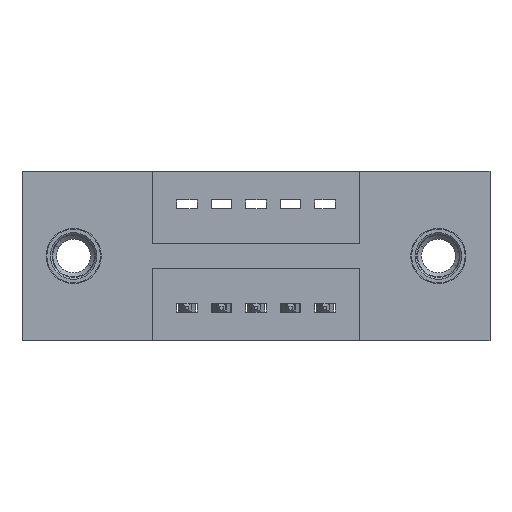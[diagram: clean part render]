
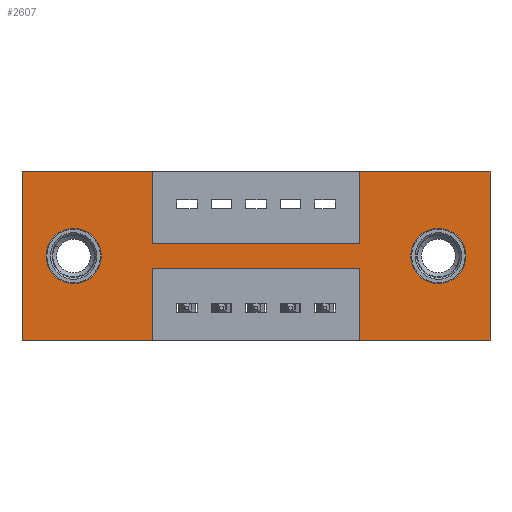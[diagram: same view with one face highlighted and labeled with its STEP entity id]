
A CAD part, front view. The second image highlights one B-rep face of the part: STEP entity #2607.
In plain terms, the highlighted planar face has unit normal (0, -1, 0).
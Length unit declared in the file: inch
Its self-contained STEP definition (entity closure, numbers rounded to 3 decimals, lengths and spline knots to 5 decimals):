
#157 = CARTESIAN_POINT ( 'NONE',  ( 0.1495, 0., -0.245 ) ) ;
#197 = DIRECTION ( 'NONE',  ( 1., 0., 0. ) ) ;
#203 = AXIS2_PLACEMENT_3D ( 'NONE', #157, #5057, #3657 ) ;
#248 = VECTOR ( 'NONE', #7604, 39.37008 ) ;
#286 = DIRECTION ( 'NONE',  ( 0., 0., -1. ) ) ;
#350 = EDGE_LOOP ( 'NONE', ( #7733, #8435, #835, #699, #1627, #6463, #6455, #4688, #6241, #8505, #3470, #5362 ) ) ;
#413 = EDGE_CURVE ( 'NONE', #2825, #4843, #7675, .T. ) ;
#619 = CARTESIAN_POINT ( 'NONE',  ( 0.3775, 0., -0.21 ) ) ;
#699 = ORIENTED_EDGE ( 'NONE', *, *, #1293, .F. ) ;
#725 = CARTESIAN_POINT ( 'NONE',  ( 0.3775, 0., -0.28 ) ) ;
#753 = CARTESIAN_POINT ( 'NONE',  ( 0., 0., 0. ) ) ;
#770 = DIRECTION ( 'NONE',  ( 0., 0., 1. ) ) ;
#835 = ORIENTED_EDGE ( 'NONE', *, *, #8266, .F. ) ;
#943 = DIRECTION ( 'NONE',  ( 0., 0., -1. ) ) ;
#1012 = VECTOR ( 'NONE', #1283, 39.37008 ) ;
#1149 = ORIENTED_EDGE ( 'NONE', *, *, #6094, .T. ) ;
#1283 = DIRECTION ( 'NONE',  ( 0., 0., -1. ) ) ;
#1293 = EDGE_CURVE ( 'NONE', #7186, #2283, #7111, .T. ) ;
#1465 = CIRCLE ( 'NONE', #5877, 0.08 ) ;
#1468 = FACE_BOUND ( 'NONE', #7034, .T. ) ;
#1577 = VERTEX_POINT ( 'NONE', #7844 ) ;
#1581 = FACE_BOUND ( 'NONE', #3711, .T. ) ;
#1608 = CARTESIAN_POINT ( 'NONE',  ( 0.3775, 0., 0. ) ) ;
#1627 = ORIENTED_EDGE ( 'NONE', *, *, #3113, .F. ) ;
#1644 = LINE ( 'NONE', #619, #4049 ) ;
#1812 = VECTOR ( 'NONE', #197, 39.37008 ) ;
#1910 = VECTOR ( 'NONE', #5036, 39.37008 ) ;
#1930 = AXIS2_PLACEMENT_3D ( 'NONE', #2100, #3488, #770 ) ;
#2018 = CARTESIAN_POINT ( 'NONE',  ( 1.2055, 0., -0.165 ) ) ;
#2030 = CARTESIAN_POINT ( 'NONE',  ( 0.9775, 0., -0.21 ) ) ;
#2049 = DIRECTION ( 'NONE',  ( 0., 0., -1. ) ) ;
#2100 = CARTESIAN_POINT ( 'NONE',  ( 0.1495, 0., -0.245 ) ) ;
#2242 = VECTOR ( 'NONE', #4327, 39.37008 ) ;
#2283 = VERTEX_POINT ( 'NONE', #1608 ) ;
#2378 = DIRECTION ( 'NONE',  ( 0., 0., 1. ) ) ;
#2573 = LINE ( 'NONE', #725, #2242 ) ;
#2589 = EDGE_CURVE ( 'NONE', #6761, #2830, #4214, .T. ) ;
#2607 = ADVANCED_FACE ( 'NONE', ( #1468, #1581, #5552 ), #3781, .T. ) ;
#2649 = VECTOR ( 'NONE', #5349, 39.37008 ) ;
#2789 = CARTESIAN_POINT ( 'NONE',  ( 0.1495, 0., -0.165 ) ) ;
#2804 = DIRECTION ( 'NONE',  ( -1., 0., 0. ) ) ;
#2825 = VERTEX_POINT ( 'NONE', #8966 ) ;
#2830 = VERTEX_POINT ( 'NONE', #4775 ) ;
#2859 = LINE ( 'NONE', #6645, #8335 ) ;
#2937 = CARTESIAN_POINT ( 'NONE',  ( 1.2055, 0., -0.325 ) ) ;
#2944 = EDGE_CURVE ( 'NONE', #4843, #2825, #4205, .T. ) ;
#2997 = VERTEX_POINT ( 'NONE', #4907 ) ;
#3080 = VECTOR ( 'NONE', #3163, 39.37008 ) ;
#3113 = EDGE_CURVE ( 'NONE', #1577, #7186, #7247, .T. ) ;
#3115 = CARTESIAN_POINT ( 'NONE',  ( 0.3775, 0., -0.21 ) ) ;
#3122 = CARTESIAN_POINT ( 'NONE',  ( 0.9775, 0., 0. ) ) ;
#3163 = DIRECTION ( 'NONE',  ( -1., 0., 0. ) ) ;
#3470 = ORIENTED_EDGE ( 'NONE', *, *, #3805, .F. ) ;
#3488 = DIRECTION ( 'NONE',  ( 0., 1., 0. ) ) ;
#3498 = EDGE_CURVE ( 'NONE', #4515, #8754, #4322, .T. ) ;
#3640 = CARTESIAN_POINT ( 'NONE',  ( 0.3775, 0., -0.49 ) ) ;
#3649 = CARTESIAN_POINT ( 'NONE',  ( 1.355, 0., 0. ) ) ;
#3657 = DIRECTION ( 'NONE',  ( 0., 0., 1. ) ) ;
#3690 = EDGE_CURVE ( 'NONE', #2997, #7426, #2573, .T. ) ;
#3711 = EDGE_LOOP ( 'NONE', ( #3800, #4841 ) ) ;
#3759 = CIRCLE ( 'NONE', #8379, 0.08 ) ;
#3781 = PLANE ( 'NONE',  #7533 ) ;
#3800 = ORIENTED_EDGE ( 'NONE', *, *, #2944, .T. ) ;
#3805 = EDGE_CURVE ( 'NONE', #8754, #5808, #9011, .T. ) ;
#4028 = CARTESIAN_POINT ( 'NONE',  ( 0.9775, 0., -0.49 ) ) ;
#4033 = EDGE_CURVE ( 'NONE', #6139, #8283, #3759, .T. ) ;
#4049 = VECTOR ( 'NONE', #7643, 39.37008 ) ;
#4069 = VECTOR ( 'NONE', #2804, 39.37008 ) ;
#4129 = EDGE_CURVE ( 'NONE', #2830, #4515, #6167, .T. ) ;
#4205 = CIRCLE ( 'NONE', #1930, 0.08 ) ;
#4214 = LINE ( 'NONE', #5233, #1812 ) ;
#4322 = LINE ( 'NONE', #4765, #8571 ) ;
#4327 = DIRECTION ( 'NONE',  ( -1., 0., 0. ) ) ;
#4515 = VERTEX_POINT ( 'NONE', #3122 ) ;
#4688 = ORIENTED_EDGE ( 'NONE', *, *, #3690, .F. ) ;
#4765 = CARTESIAN_POINT ( 'NONE',  ( 0., 0., 0. ) ) ;
#4775 = CARTESIAN_POINT ( 'NONE',  ( 0.9775, 0., -0.21 ) ) ;
#4841 = ORIENTED_EDGE ( 'NONE', *, *, #413, .T. ) ;
#4843 = VERTEX_POINT ( 'NONE', #2789 ) ;
#4907 = CARTESIAN_POINT ( 'NONE',  ( 0.9775, 0., -0.28 ) ) ;
#4957 = LINE ( 'NONE', #8681, #3080 ) ;
#4972 = EDGE_CURVE ( 'NONE', #5808, #8410, #7332, .T. ) ;
#5036 = DIRECTION ( 'NONE',  ( 0., 0., 1. ) ) ;
#5057 = DIRECTION ( 'NONE',  ( 0., 1., 0. ) ) ;
#5233 = CARTESIAN_POINT ( 'NONE',  ( 0.3775, 0., -0.21 ) ) ;
#5312 = VECTOR ( 'NONE', #943, 39.37008 ) ;
#5349 = DIRECTION ( 'NONE',  ( 1., 0., 0. ) ) ;
#5362 = ORIENTED_EDGE ( 'NONE', *, *, #3498, .F. ) ;
#5378 = CARTESIAN_POINT ( 'NONE',  ( 0., 0., 0. ) ) ;
#5457 = CARTESIAN_POINT ( 'NONE',  ( 1.2055, 0., -0.245 ) ) ;
#5552 = FACE_OUTER_BOUND ( 'NONE', #350, .T. ) ;
#5719 = LINE ( 'NONE', #6855, #1012 ) ;
#5769 = CARTESIAN_POINT ( 'NONE',  ( 1.2055, 0., -0.245 ) ) ;
#5808 = VERTEX_POINT ( 'NONE', #7603 ) ;
#5877 = AXIS2_PLACEMENT_3D ( 'NONE', #5769, #8545, #8597 ) ;
#6094 = EDGE_CURVE ( 'NONE', #8283, #6139, #1465, .T. ) ;
#6139 = VERTEX_POINT ( 'NONE', #2937 ) ;
#6167 = LINE ( 'NONE', #2030, #248 ) ;
#6241 = ORIENTED_EDGE ( 'NONE', *, *, #8796, .F. ) ;
#6242 = DIRECTION ( 'NONE',  ( 1., 0., 0. ) ) ;
#6310 = CARTESIAN_POINT ( 'NONE',  ( 0., 0., -0.49 ) ) ;
#6455 = ORIENTED_EDGE ( 'NONE', *, *, #7073, .F. ) ;
#6460 = CARTESIAN_POINT ( 'NONE',  ( 0., 0., 0. ) ) ;
#6463 = ORIENTED_EDGE ( 'NONE', *, *, #7377, .F. ) ;
#6569 = CARTESIAN_POINT ( 'NONE',  ( 1.355, 0., 0. ) ) ;
#6645 = CARTESIAN_POINT ( 'NONE',  ( 0.9775, 0., -0.28 ) ) ;
#6692 = VERTEX_POINT ( 'NONE', #3640 ) ;
#6761 = VERTEX_POINT ( 'NONE', #3115 ) ;
#6855 = CARTESIAN_POINT ( 'NONE',  ( 0.3775, 0., -0.28 ) ) ;
#7034 = EDGE_LOOP ( 'NONE', ( #1149, #8295 ) ) ;
#7073 = EDGE_CURVE ( 'NONE', #7426, #6692, #5719, .T. ) ;
#7111 = LINE ( 'NONE', #5378, #2649 ) ;
#7186 = VERTEX_POINT ( 'NONE', #753 ) ;
#7247 = LINE ( 'NONE', #6460, #1910 ) ;
#7312 = CARTESIAN_POINT ( 'NONE',  ( 0., 0., -0.49 ) ) ;
#7332 = LINE ( 'NONE', #6310, #4069 ) ;
#7377 = EDGE_CURVE ( 'NONE', #6692, #1577, #4957, .T. ) ;
#7426 = VERTEX_POINT ( 'NONE', #8849 ) ;
#7533 = AXIS2_PLACEMENT_3D ( 'NONE', #7312, #8031, #286 ) ;
#7603 = CARTESIAN_POINT ( 'NONE',  ( 1.355, 0., -0.49 ) ) ;
#7604 = DIRECTION ( 'NONE',  ( 0., 0., 1. ) ) ;
#7643 = DIRECTION ( 'NONE',  ( 0., 0., -1. ) ) ;
#7675 = CIRCLE ( 'NONE', #203, 0.08 ) ;
#7733 = ORIENTED_EDGE ( 'NONE', *, *, #4129, .F. ) ;
#7844 = CARTESIAN_POINT ( 'NONE',  ( 0., 0., -0.49 ) ) ;
#8031 = DIRECTION ( 'NONE',  ( 0., -1., 0. ) ) ;
#8266 = EDGE_CURVE ( 'NONE', #2283, #6761, #1644, .T. ) ;
#8283 = VERTEX_POINT ( 'NONE', #2018 ) ;
#8295 = ORIENTED_EDGE ( 'NONE', *, *, #4033, .T. ) ;
#8335 = VECTOR ( 'NONE', #2378, 39.37008 ) ;
#8379 = AXIS2_PLACEMENT_3D ( 'NONE', #5457, #9013, #2049 ) ;
#8410 = VERTEX_POINT ( 'NONE', #4028 ) ;
#8435 = ORIENTED_EDGE ( 'NONE', *, *, #2589, .F. ) ;
#8505 = ORIENTED_EDGE ( 'NONE', *, *, #4972, .F. ) ;
#8545 = DIRECTION ( 'NONE',  ( 0., 1., 0. ) ) ;
#8571 = VECTOR ( 'NONE', #6242, 39.37008 ) ;
#8597 = DIRECTION ( 'NONE',  ( 0., 0., -1. ) ) ;
#8681 = CARTESIAN_POINT ( 'NONE',  ( 0., 0., -0.49 ) ) ;
#8754 = VERTEX_POINT ( 'NONE', #3649 ) ;
#8796 = EDGE_CURVE ( 'NONE', #8410, #2997, #2859, .T. ) ;
#8849 = CARTESIAN_POINT ( 'NONE',  ( 0.3775, 0., -0.28 ) ) ;
#8966 = CARTESIAN_POINT ( 'NONE',  ( 0.1495, 0., -0.325 ) ) ;
#9011 = LINE ( 'NONE', #6569, #5312 ) ;
#9013 = DIRECTION ( 'NONE',  ( 0., 1., 0. ) ) ;
